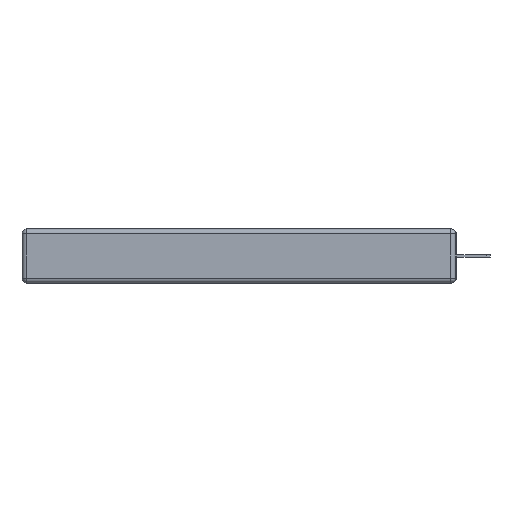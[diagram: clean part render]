
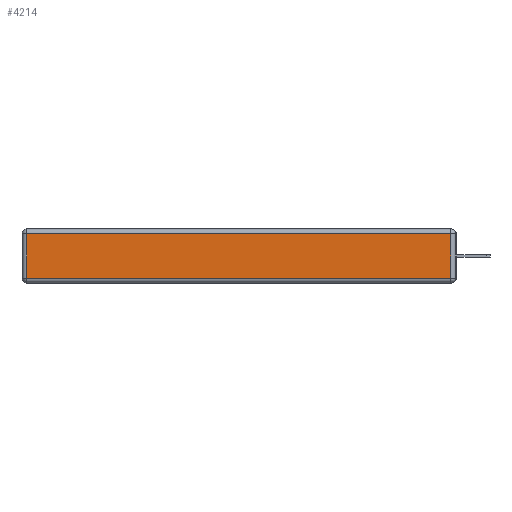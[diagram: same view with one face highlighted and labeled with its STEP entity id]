
A CAD part, left-side view. The second image highlights one B-rep face of the part: STEP entity #4214.
In plain terms, the highlighted planar face has unit normal (-1, 0, 0).
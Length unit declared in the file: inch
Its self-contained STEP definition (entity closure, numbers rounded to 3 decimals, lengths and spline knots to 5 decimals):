
#659 = EDGE_CURVE ( 'NONE', #12789, #12759, #11814, .T. ) ;
#661 = EDGE_CURVE ( 'NONE', #12759, #13723, #9394, .T. ) ;
#686 = EDGE_CURVE ( 'NONE', #13723, #8617, #13858, .T. ) ;
#690 = EDGE_CURVE ( 'NONE', #8617, #12789, #2604, .T. ) ;
#1311 = AXIS2_PLACEMENT_3D ( 'NONE', #8883, #10994, #4518 ) ;
#2604 = LINE ( 'NONE', #11417, #10847 ) ;
#3248 = PLANE ( 'NONE',  #1311 ) ;
#4214 = ADVANCED_FACE ( 'NONE', ( #13026 ), #3248, .T. ) ;
#4518 = DIRECTION ( 'NONE',  ( 0., 0., 1. ) ) ;
#5012 = DIRECTION ( 'NONE',  ( 0., 0., -1. ) ) ;
#5351 = EDGE_LOOP ( 'NONE', ( #7167, #9201, #7108, #8386 ) ) ;
#6745 = CARTESIAN_POINT ( 'NONE',  ( 0., 2.72, -0.313 ) ) ;
#7108 = ORIENTED_EDGE ( 'NONE', *, *, #686, .T. ) ;
#7167 = ORIENTED_EDGE ( 'NONE', *, *, #659, .T. ) ;
#7204 = CARTESIAN_POINT ( 'NONE',  ( 0., 2.75, -0.03 ) ) ;
#7824 = CARTESIAN_POINT ( 'NONE',  ( 0., 0.03, -0.313 ) ) ;
#8241 = DIRECTION ( 'NONE',  ( 0., 1., 0. ) ) ;
#8386 = ORIENTED_EDGE ( 'NONE', *, *, #690, .T. ) ;
#8420 = DIRECTION ( 'NONE',  ( 0., -1., 0. ) ) ;
#8617 = VERTEX_POINT ( 'NONE', #9034 ) ;
#8883 = CARTESIAN_POINT ( 'NONE',  ( 0., 0., -0.343 ) ) ;
#9034 = CARTESIAN_POINT ( 'NONE',  ( 0., 2.72, -0.03 ) ) ;
#9064 = VECTOR ( 'NONE', #8420, 39.37008 ) ;
#9201 = ORIENTED_EDGE ( 'NONE', *, *, #661, .T. ) ;
#9394 = LINE ( 'NONE', #10285, #14182 ) ;
#10285 = CARTESIAN_POINT ( 'NONE',  ( 0., 0.03, -0.343 ) ) ;
#10545 = DIRECTION ( 'NONE',  ( 0., 0., 1. ) ) ;
#10847 = VECTOR ( 'NONE', #5012, 39.37008 ) ;
#10994 = DIRECTION ( 'NONE',  ( -1., 0., 0. ) ) ;
#11417 = CARTESIAN_POINT ( 'NONE',  ( 0., 2.72, -0.343 ) ) ;
#11508 = VECTOR ( 'NONE', #8241, 39.37008 ) ;
#11814 = LINE ( 'NONE', #14312, #9064 ) ;
#12061 = CARTESIAN_POINT ( 'NONE',  ( 0., 0.03, -0.03 ) ) ;
#12759 = VERTEX_POINT ( 'NONE', #7824 ) ;
#12789 = VERTEX_POINT ( 'NONE', #6745 ) ;
#13026 = FACE_OUTER_BOUND ( 'NONE', #5351, .T. ) ;
#13723 = VERTEX_POINT ( 'NONE', #12061 ) ;
#13858 = LINE ( 'NONE', #7204, #11508 ) ;
#14182 = VECTOR ( 'NONE', #10545, 39.37008 ) ;
#14312 = CARTESIAN_POINT ( 'NONE',  ( 0., 0., -0.313 ) ) ;
